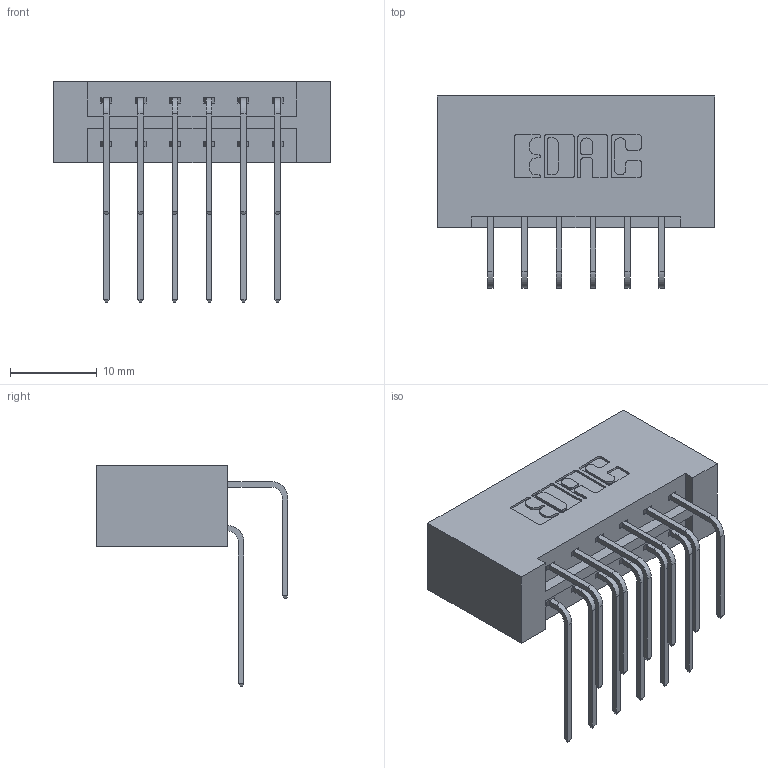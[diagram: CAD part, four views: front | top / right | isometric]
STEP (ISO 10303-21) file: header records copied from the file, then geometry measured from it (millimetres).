
FILE_DESCRIPTION (( 'STEP AP203' ), '1' );
FILE_NAME ('333-012-558-201.STEP', '2018-08-01T00:48:54', ( '' ), ( '' ), 'SwSTEP 2.0', 'SolidWorks 2016', '' );
FILE_SCHEMA (( 'CONFIG_CONTROL_DESIGN' ));
Length unit declared in the file: inch
Products named in the file (4): 345-292-001_558 559 Tail - 1; 345-292-001_558 Tail - 2; 333-012-558-201; 333 Part_Lugless
Assembly tree (13 placements, depth 2):
  333-012-558-201
    333 Part_Lugless
    345-292-001_558 559 Tail - 1  x6
    345-292-001_558 Tail - 2  x6
Bounding box: 32.03 x 22.17 x 25.53 mm (x, y, z)
Volume: 3634.8 mm3; surface area: 4279.6 mm2
Topology: 13 solids, 13 shells, 754 faces, 2219 edges, 1462 vertices
Faces by surface type: plane 522, cylinder 232
Entity records: 10023 total; most frequent: CARTESIAN_POINT 1753, ORIENTED_EDGE 1638, DIRECTION 1535, EDGE_CURVE 819, LINE 659, VECTOR 659, VERTEX_POINT 542, AXIS2_PLACEMENT_3D 438
